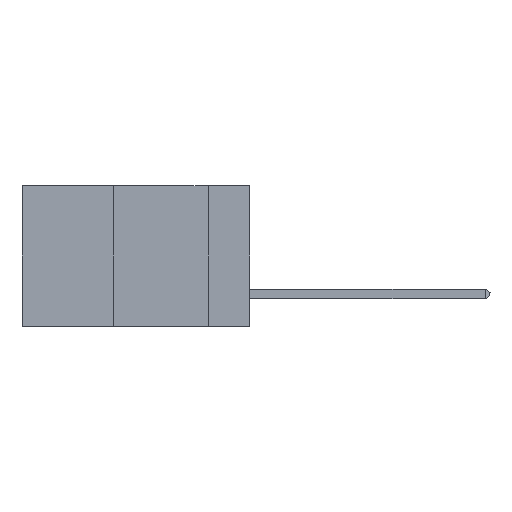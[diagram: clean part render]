
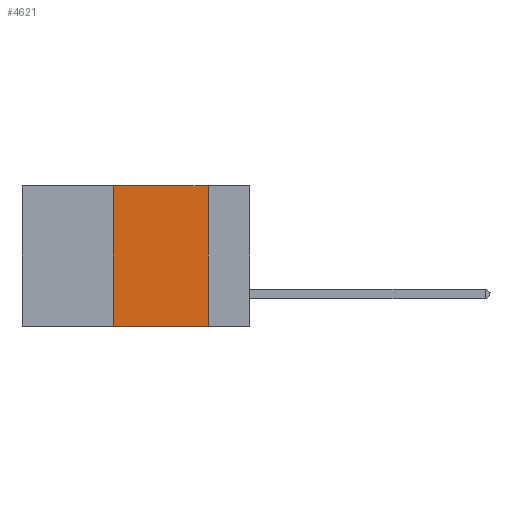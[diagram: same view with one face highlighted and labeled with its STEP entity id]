
A CAD part, left-side view. The second image highlights one B-rep face of the part: STEP entity #4621.
In plain terms, the highlighted planar face has unit normal (-1, 0, 0).
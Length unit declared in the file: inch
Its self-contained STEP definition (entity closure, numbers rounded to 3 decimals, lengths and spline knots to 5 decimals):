
#575 = CARTESIAN_POINT ( 'NONE',  ( 0., 0.6, -0.37 ) ) ;
#704 = VECTOR ( 'NONE', #15298, 39.37008 ) ;
#4621 = ADVANCED_FACE ( 'NONE', ( #11394 ), #24892, .F. ) ;
#5021 = LINE ( 'NONE', #5749, #24918 ) ;
#5749 = CARTESIAN_POINT ( 'NONE',  ( 0., 0.6, 0. ) ) ;
#6023 = VERTEX_POINT ( 'NONE', #25189 ) ;
#8271 = CARTESIAN_POINT ( 'NONE',  ( 0., 0.36, 0. ) ) ;
#8299 = EDGE_LOOP ( 'NONE', ( #21826, #24582, #19345, #28515 ) ) ;
#8347 = EDGE_CURVE ( 'NONE', #25182, #18818, #13690, .T. ) ;
#8970 = VECTOR ( 'NONE', #16662, 39.37008 ) ;
#10787 = CARTESIAN_POINT ( 'NONE',  ( 0., 0.36, 0. ) ) ;
#11394 = FACE_OUTER_BOUND ( 'NONE', #8299, .T. ) ;
#12027 = VERTEX_POINT ( 'NONE', #20555 ) ;
#13391 = CARTESIAN_POINT ( 'NONE',  ( 0., 0.6, 0. ) ) ;
#13690 = LINE ( 'NONE', #8271, #704 ) ;
#15298 = DIRECTION ( 'NONE',  ( 0., 0., 1. ) ) ;
#15391 = LINE ( 'NONE', #17712, #24806 ) ;
#16158 = EDGE_CURVE ( 'NONE', #25182, #6023, #28069, .T. ) ;
#16662 = DIRECTION ( 'NONE',  ( 0., -1., 0. ) ) ;
#17712 = CARTESIAN_POINT ( 'NONE',  ( 0., 0.11, 0. ) ) ;
#17869 = AXIS2_PLACEMENT_3D ( 'NONE', #13391, #27429, #18040 ) ;
#18040 = DIRECTION ( 'NONE',  ( 0., 0., -1. ) ) ;
#18818 = VERTEX_POINT ( 'NONE', #10787 ) ;
#19345 = ORIENTED_EDGE ( 'NONE', *, *, #8347, .F. ) ;
#19657 = DIRECTION ( 'NONE',  ( 0., -1., 0. ) ) ;
#20555 = CARTESIAN_POINT ( 'NONE',  ( 0., 0.11, 0. ) ) ;
#21826 = ORIENTED_EDGE ( 'NONE', *, *, #28536, .F. ) ;
#23781 = EDGE_CURVE ( 'NONE', #18818, #12027, #5021, .T. ) ;
#24582 = ORIENTED_EDGE ( 'NONE', *, *, #23781, .F. ) ;
#24806 = VECTOR ( 'NONE', #24970, 39.37008 ) ;
#24892 = PLANE ( 'NONE',  #17869 ) ;
#24918 = VECTOR ( 'NONE', #19657, 39.37008 ) ;
#24970 = DIRECTION ( 'NONE',  ( 0., 0., -1. ) ) ;
#25182 = VERTEX_POINT ( 'NONE', #26757 ) ;
#25189 = CARTESIAN_POINT ( 'NONE',  ( 0., 0.11, -0.37 ) ) ;
#26757 = CARTESIAN_POINT ( 'NONE',  ( 0., 0.36, -0.37 ) ) ;
#27429 = DIRECTION ( 'NONE',  ( 1., 0., 0. ) ) ;
#28069 = LINE ( 'NONE', #575, #8970 ) ;
#28515 = ORIENTED_EDGE ( 'NONE', *, *, #16158, .T. ) ;
#28536 = EDGE_CURVE ( 'NONE', #12027, #6023, #15391, .T. ) ;
